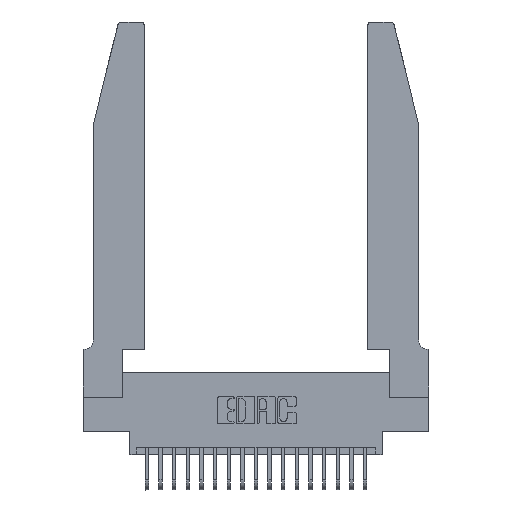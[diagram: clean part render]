
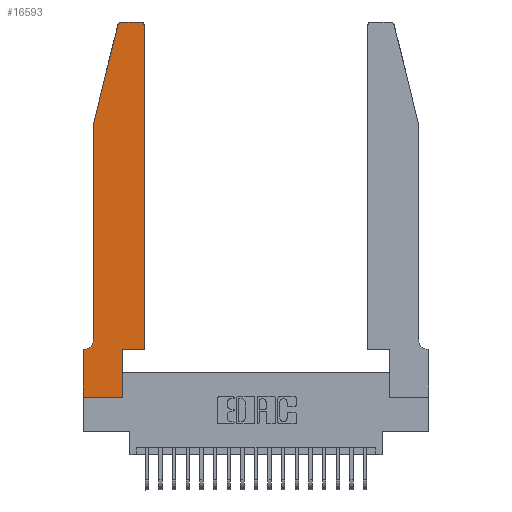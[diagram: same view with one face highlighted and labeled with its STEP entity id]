
A CAD part, top view. The second image highlights one B-rep face of the part: STEP entity #16593.
In plain terms, the highlighted planar face has unit normal (0, 0, 1).
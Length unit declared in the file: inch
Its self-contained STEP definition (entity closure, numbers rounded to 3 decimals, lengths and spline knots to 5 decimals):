
#322 = EDGE_LOOP ( 'NONE', ( #2352, #1047, #2474, #14704, #16754, #20043, #1885, #3793, #3684, #1485, #14431, #3720 ) ) ;
#463 = VERTEX_POINT ( 'NONE', #6909 ) ;
#513 = LINE ( 'NONE', #3324, #21157 ) ;
#557 = EDGE_CURVE ( 'NONE', #11072, #5754, #12803, .T. ) ;
#651 = CARTESIAN_POINT ( 'NONE',  ( 0.2865, 0., 0.37 ) ) ;
#1047 = ORIENTED_EDGE ( 'NONE', *, *, #7209, .T. ) ;
#1485 = ORIENTED_EDGE ( 'NONE', *, *, #17957, .T. ) ;
#1696 = CARTESIAN_POINT ( 'NONE',  ( 0.4505, 0.35, 0.37 ) ) ;
#1885 = ORIENTED_EDGE ( 'NONE', *, *, #18374, .T. ) ;
#1955 = EDGE_CURVE ( 'NONE', #5754, #6668, #17539, .T. ) ;
#2072 = AXIS2_PLACEMENT_3D ( 'NONE', #18012, #8381, #19619 ) ;
#2352 = ORIENTED_EDGE ( 'NONE', *, *, #13162, .T. ) ;
#2474 = ORIENTED_EDGE ( 'NONE', *, *, #13004, .T. ) ;
#2698 = LINE ( 'NONE', #20356, #10917 ) ;
#3023 = CARTESIAN_POINT ( 'NONE',  ( 0.4205, 2.75, 0.37 ) ) ;
#3025 = CARTESIAN_POINT ( 'NONE',  ( 0.284, 2.75, 0.37 ) ) ;
#3324 = CARTESIAN_POINT ( 'NONE',  ( 0.2865, 0.35, 0.37 ) ) ;
#3575 = VECTOR ( 'NONE', #20237, 39.37008 ) ;
#3684 = ORIENTED_EDGE ( 'NONE', *, *, #12421, .T. ) ;
#3720 = ORIENTED_EDGE ( 'NONE', *, *, #9736, .T. ) ;
#3793 = ORIENTED_EDGE ( 'NONE', *, *, #12627, .T. ) ;
#3893 = CARTESIAN_POINT ( 'NONE',  ( 0., 0., 0.37 ) ) ;
#4761 = DIRECTION ( 'NONE',  ( -0.239, -0.971, 0. ) ) ;
#4936 = CARTESIAN_POINT ( 'NONE',  ( 0.4205, 2.72, 0.37 ) ) ;
#5267 = LINE ( 'NONE', #8801, #18187 ) ;
#5520 = CARTESIAN_POINT ( 'NONE',  ( 0.2865, 0.35, 0.37 ) ) ;
#5754 = VERTEX_POINT ( 'NONE', #7504 ) ;
#5785 = AXIS2_PLACEMENT_3D ( 'NONE', #4936, #16268, #6614 ) ;
#5898 = VECTOR ( 'NONE', #14262, 39.37008 ) ;
#5957 = DIRECTION ( 'NONE',  ( -1., 0., 0. ) ) ;
#5988 = DIRECTION ( 'NONE',  ( 0., 0., -1. ) ) ;
#5993 = CARTESIAN_POINT ( 'NONE',  ( 0.0055, 0.42, 0.37 ) ) ;
#6430 = CARTESIAN_POINT ( 'NONE',  ( 0.4505, 0.35, 0.37 ) ) ;
#6585 = AXIS2_PLACEMENT_3D ( 'NONE', #19406, #9767, #20976 ) ;
#6614 = DIRECTION ( 'NONE',  ( 1., 0., 0. ) ) ;
#6668 = VERTEX_POINT ( 'NONE', #19286 ) ;
#6734 = PLANE ( 'NONE',  #2072 ) ;
#6786 = CARTESIAN_POINT ( 'NONE',  ( 0.0755, 0.42, 0.37 ) ) ;
#6796 = DIRECTION ( 'NONE',  ( -1., 0., 0. ) ) ;
#6909 = CARTESIAN_POINT ( 'NONE',  ( 0.0755, 2., 0.37 ) ) ;
#7209 = EDGE_CURVE ( 'NONE', #19258, #13975, #19719, .T. ) ;
#7339 = CARTESIAN_POINT ( 'NONE',  ( 0.4505, 0.35, 0.37 ) ) ;
#7355 = LINE ( 'NONE', #11231, #15894 ) ;
#7504 = CARTESIAN_POINT ( 'NONE',  ( 0.0055, 0.35, 0.37 ) ) ;
#7992 = VERTEX_POINT ( 'NONE', #651 ) ;
#8381 = DIRECTION ( 'NONE',  ( 0., 0., 1. ) ) ;
#8801 = CARTESIAN_POINT ( 'NONE',  ( 0., 0., 0.37 ) ) ;
#9330 = CARTESIAN_POINT ( 'NONE',  ( 0.25487, 2.72718, 0.37 ) ) ;
#9331 = CARTESIAN_POINT ( 'NONE',  ( 0.4505, 2.72, 0.37 ) ) ;
#9736 = EDGE_CURVE ( 'NONE', #15887, #20117, #12315, .T. ) ;
#9767 = DIRECTION ( 'NONE',  ( 0., 0., 1. ) ) ;
#10228 = LINE ( 'NONE', #17460, #5898 ) ;
#10632 = VECTOR ( 'NONE', #11362, 39.37008 ) ;
#10917 = VECTOR ( 'NONE', #15583, 39.37008 ) ;
#11072 = VERTEX_POINT ( 'NONE', #6786 ) ;
#11231 = CARTESIAN_POINT ( 'NONE',  ( 0.0755, 2., 0.37 ) ) ;
#11362 = DIRECTION ( 'NONE',  ( 1., 0., 0. ) ) ;
#12230 = LINE ( 'NONE', #7339, #3575 ) ;
#12315 = CIRCLE ( 'NONE', #5785, 0.03 ) ;
#12421 = EDGE_CURVE ( 'NONE', #7992, #18913, #513, .T. ) ;
#12627 = EDGE_CURVE ( 'NONE', #15094, #7992, #5267, .T. ) ;
#12803 = CIRCLE ( 'NONE', #21041, 0.07 ) ;
#12858 = LINE ( 'NONE', #19677, #20884 ) ;
#13004 = EDGE_CURVE ( 'NONE', #13975, #463, #7355, .T. ) ;
#13109 = CARTESIAN_POINT ( 'NONE',  ( 0.0755, 0.35, 0.37 ) ) ;
#13162 = EDGE_CURVE ( 'NONE', #20117, #19258, #12858, .T. ) ;
#13975 = VERTEX_POINT ( 'NONE', #9330 ) ;
#14262 = DIRECTION ( 'NONE',  ( 0., -1., 0. ) ) ;
#14274 = VERTEX_POINT ( 'NONE', #1696 ) ;
#14431 = ORIENTED_EDGE ( 'NONE', *, *, #19543, .T. ) ;
#14704 = ORIENTED_EDGE ( 'NONE', *, *, #19671, .T. ) ;
#14910 = LINE ( 'NONE', #6430, #10632 ) ;
#15094 = VERTEX_POINT ( 'NONE', #3893 ) ;
#15171 = DIRECTION ( 'NONE',  ( 1., 0., 0. ) ) ;
#15583 = DIRECTION ( 'NONE',  ( 0., -1., 0. ) ) ;
#15887 = VERTEX_POINT ( 'NONE', #9331 ) ;
#15894 = VECTOR ( 'NONE', #4761, 39.37008 ) ;
#16268 = DIRECTION ( 'NONE',  ( 0., 0., 1. ) ) ;
#16593 = ADVANCED_FACE ( 'NONE', ( #19755 ), #6734, .T. ) ;
#16754 = ORIENTED_EDGE ( 'NONE', *, *, #557, .T. ) ;
#17033 = VECTOR ( 'NONE', #18821, 39.37008 ) ;
#17460 = CARTESIAN_POINT ( 'NONE',  ( 0.0755, 2., 0.37 ) ) ;
#17539 = LINE ( 'NONE', #13109, #17033 ) ;
#17957 = EDGE_CURVE ( 'NONE', #18913, #14274, #14910, .T. ) ;
#18012 = CARTESIAN_POINT ( 'NONE',  ( 0., 0.35, 0.37 ) ) ;
#18187 = VECTOR ( 'NONE', #15171, 39.37008 ) ;
#18374 = EDGE_CURVE ( 'NONE', #6668, #15094, #2698, .T. ) ;
#18821 = DIRECTION ( 'NONE',  ( -1., 0., 0. ) ) ;
#18913 = VERTEX_POINT ( 'NONE', #5520 ) ;
#19258 = VERTEX_POINT ( 'NONE', #3025 ) ;
#19286 = CARTESIAN_POINT ( 'NONE',  ( 0., 0.35, 0.37 ) ) ;
#19406 = CARTESIAN_POINT ( 'NONE',  ( 0.284, 2.72, 0.37 ) ) ;
#19543 = EDGE_CURVE ( 'NONE', #14274, #15887, #12230, .T. ) ;
#19619 = DIRECTION ( 'NONE',  ( 1., 0., 0. ) ) ;
#19671 = EDGE_CURVE ( 'NONE', #463, #11072, #10228, .T. ) ;
#19677 = CARTESIAN_POINT ( 'NONE',  ( 0.2605, 2.75, 0.37 ) ) ;
#19719 = CIRCLE ( 'NONE', #6585, 0.03 ) ;
#19755 = FACE_OUTER_BOUND ( 'NONE', #322, .T. ) ;
#20043 = ORIENTED_EDGE ( 'NONE', *, *, #1955, .T. ) ;
#20117 = VERTEX_POINT ( 'NONE', #3023 ) ;
#20237 = DIRECTION ( 'NONE',  ( 0., 1., 0. ) ) ;
#20356 = CARTESIAN_POINT ( 'NONE',  ( 0., 0., 0.37 ) ) ;
#20884 = VECTOR ( 'NONE', #6796, 39.37008 ) ;
#20976 = DIRECTION ( 'NONE',  ( 1., 0., 0. ) ) ;
#21041 = AXIS2_PLACEMENT_3D ( 'NONE', #5993, #5988, #5957 ) ;
#21069 = DIRECTION ( 'NONE',  ( 0., 1., 0. ) ) ;
#21157 = VECTOR ( 'NONE', #21069, 39.37008 ) ;
